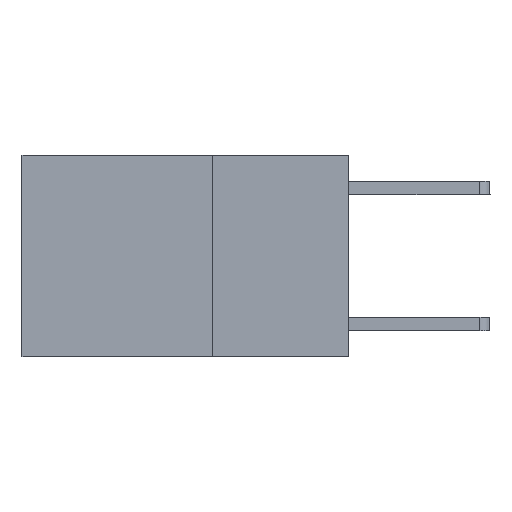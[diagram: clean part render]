
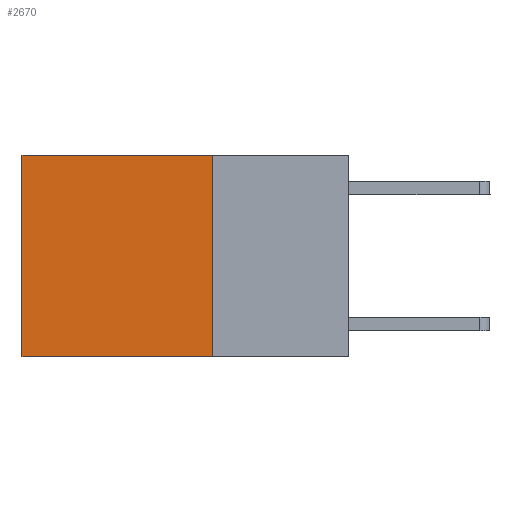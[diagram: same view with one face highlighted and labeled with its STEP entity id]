
A CAD part, left-side view. The second image highlights one B-rep face of the part: STEP entity #2670.
In plain terms, the highlighted planar face has unit normal (-1, 0, 0).
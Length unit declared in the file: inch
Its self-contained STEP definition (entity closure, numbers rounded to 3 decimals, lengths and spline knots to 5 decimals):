
#48 = ORIENTED_EDGE ( 'NONE', *, *, #3712, .T. ) ;
#165 = DIRECTION ( 'NONE',  ( 0., 0., -1. ) ) ;
#298 = ORIENTED_EDGE ( 'NONE', *, *, #6807, .F. ) ;
#729 = ORIENTED_EDGE ( 'NONE', *, *, #2418, .F. ) ;
#1301 = VECTOR ( 'NONE', #165, 39.37008 ) ;
#1337 = LINE ( 'NONE', #5041, #8045 ) ;
#1520 = DIRECTION ( 'NONE',  ( 0., 0., -1. ) ) ;
#2004 = VERTEX_POINT ( 'NONE', #2952 ) ;
#2418 = EDGE_CURVE ( 'NONE', #10050, #2004, #8284, .T. ) ;
#2670 = ADVANCED_FACE ( 'NONE', ( #10238 ), #5937, .F. ) ;
#2952 = CARTESIAN_POINT ( 'NONE',  ( 0.2625, 0.25, -0.37 ) ) ;
#3457 = VERTEX_POINT ( 'NONE', #9678 ) ;
#3474 = EDGE_LOOP ( 'NONE', ( #8747, #298, #729, #48 ) ) ;
#3578 = CARTESIAN_POINT ( 'NONE',  ( 0.2625, 0.6, 0. ) ) ;
#3712 = EDGE_CURVE ( 'NONE', #10050, #5586, #9440, .T. ) ;
#3822 = CARTESIAN_POINT ( 'NONE',  ( 0.2625, 0.25, 0. ) ) ;
#4106 = CARTESIAN_POINT ( 'NONE',  ( 0.2625, 0.25, 0. ) ) ;
#4929 = VECTOR ( 'NONE', #9965, 39.37008 ) ;
#5041 = CARTESIAN_POINT ( 'NONE',  ( 0.2625, 0.25, -0.37 ) ) ;
#5586 = VERTEX_POINT ( 'NONE', #6202 ) ;
#5691 = LINE ( 'NONE', #3578, #10095 ) ;
#5746 = AXIS2_PLACEMENT_3D ( 'NONE', #10704, #6794, #1520 ) ;
#5937 = PLANE ( 'NONE',  #5746 ) ;
#6202 = CARTESIAN_POINT ( 'NONE',  ( 0.2625, 0.6, 0. ) ) ;
#6794 = DIRECTION ( 'NONE',  ( 1., 0., 0. ) ) ;
#6807 = EDGE_CURVE ( 'NONE', #2004, #3457, #1337, .T. ) ;
#8045 = VECTOR ( 'NONE', #10069, 39.37008 ) ;
#8284 = LINE ( 'NONE', #3822, #1301 ) ;
#8648 = EDGE_CURVE ( 'NONE', #5586, #3457, #5691, .T. ) ;
#8694 = DIRECTION ( 'NONE',  ( 0., 0., -1. ) ) ;
#8747 = ORIENTED_EDGE ( 'NONE', *, *, #8648, .T. ) ;
#9440 = LINE ( 'NONE', #4106, #4929 ) ;
#9678 = CARTESIAN_POINT ( 'NONE',  ( 0.2625, 0.6, -0.37 ) ) ;
#9699 = CARTESIAN_POINT ( 'NONE',  ( 0.2625, 0.25, 0. ) ) ;
#9965 = DIRECTION ( 'NONE',  ( 0., 1., 0. ) ) ;
#10050 = VERTEX_POINT ( 'NONE', #9699 ) ;
#10069 = DIRECTION ( 'NONE',  ( 0., 1., 0. ) ) ;
#10095 = VECTOR ( 'NONE', #8694, 39.37008 ) ;
#10238 = FACE_OUTER_BOUND ( 'NONE', #3474, .T. ) ;
#10704 = CARTESIAN_POINT ( 'NONE',  ( 0.2625, 0.25, 0. ) ) ;
